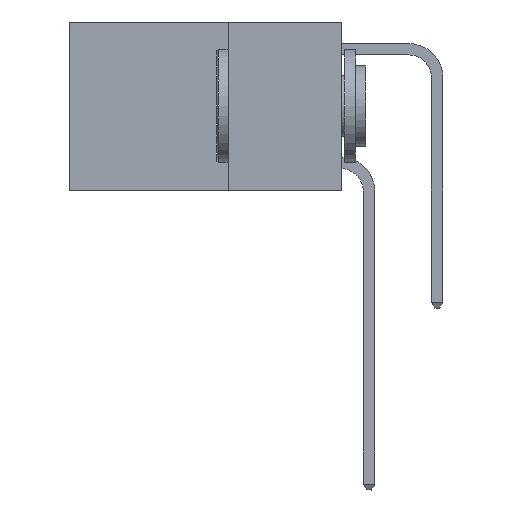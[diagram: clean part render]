
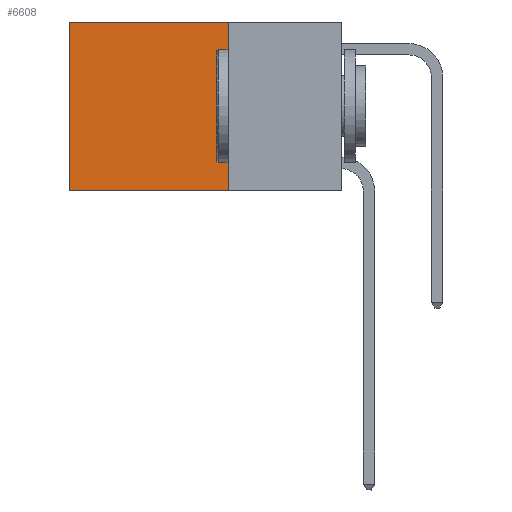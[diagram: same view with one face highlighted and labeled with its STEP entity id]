
A CAD part, left-side view. The second image highlights one B-rep face of the part: STEP entity #6608.
In plain terms, the highlighted planar face has unit normal (-1, 0, 0).
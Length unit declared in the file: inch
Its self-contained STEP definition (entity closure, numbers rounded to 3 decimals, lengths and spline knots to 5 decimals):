
#66 = CARTESIAN_POINT ( 'NONE',  ( 0.2625, 0.25, 0. ) ) ;
#132 = ORIENTED_EDGE ( 'NONE', *, *, #10196, .T. ) ;
#144 = CARTESIAN_POINT ( 'NONE',  ( 0.2625, 0.6, 0. ) ) ;
#981 = CARTESIAN_POINT ( 'NONE',  ( 0.2625, 0.6, 0. ) ) ;
#1362 = VECTOR ( 'NONE', #9491, 39.37008 ) ;
#1397 = DIRECTION ( 'NONE',  ( 1., 0., 0. ) ) ;
#1858 = VERTEX_POINT ( 'NONE', #144 ) ;
#1886 = LINE ( 'NONE', #7746, #2301 ) ;
#2301 = VECTOR ( 'NONE', #16773, 39.37008 ) ;
#2768 = CARTESIAN_POINT ( 'NONE',  ( 0.2625, 0.25, 0. ) ) ;
#4065 = LINE ( 'NONE', #981, #11034 ) ;
#4128 = ORIENTED_EDGE ( 'NONE', *, *, #5110, .F. ) ;
#5110 = EDGE_CURVE ( 'NONE', #11940, #6854, #1886, .T. ) ;
#6608 = ADVANCED_FACE ( 'NONE', ( #13193 ), #8014, .F. ) ;
#6854 = VERTEX_POINT ( 'NONE', #13717 ) ;
#7214 = ORIENTED_EDGE ( 'NONE', *, *, #8718, .F. ) ;
#7415 = CARTESIAN_POINT ( 'NONE',  ( 0.2625, 0.6, -0.37 ) ) ;
#7608 = ORIENTED_EDGE ( 'NONE', *, *, #11719, .T. ) ;
#7642 = VERTEX_POINT ( 'NONE', #7415 ) ;
#7746 = CARTESIAN_POINT ( 'NONE',  ( 0.2625, 0.25, 0. ) ) ;
#8014 = PLANE ( 'NONE',  #14003 ) ;
#8718 = EDGE_CURVE ( 'NONE', #6854, #7642, #12313, .T. ) ;
#9491 = DIRECTION ( 'NONE',  ( 0., 1., 0. ) ) ;
#10196 = EDGE_CURVE ( 'NONE', #1858, #7642, #4065, .T. ) ;
#10661 = DIRECTION ( 'NONE',  ( 0., 0., -1. ) ) ;
#11034 = VECTOR ( 'NONE', #16748, 39.37008 ) ;
#11230 = EDGE_LOOP ( 'NONE', ( #132, #7214, #4128, #7608 ) ) ;
#11602 = VECTOR ( 'NONE', #15844, 39.37008 ) ;
#11719 = EDGE_CURVE ( 'NONE', #11940, #1858, #12019, .T. ) ;
#11940 = VERTEX_POINT ( 'NONE', #16270 ) ;
#12019 = LINE ( 'NONE', #2768, #11602 ) ;
#12313 = LINE ( 'NONE', #15937, #1362 ) ;
#13193 = FACE_OUTER_BOUND ( 'NONE', #11230, .T. ) ;
#13717 = CARTESIAN_POINT ( 'NONE',  ( 0.2625, 0.25, -0.37 ) ) ;
#14003 = AXIS2_PLACEMENT_3D ( 'NONE', #66, #1397, #10661 ) ;
#15844 = DIRECTION ( 'NONE',  ( 0., 1., 0. ) ) ;
#15937 = CARTESIAN_POINT ( 'NONE',  ( 0.2625, 0.25, -0.37 ) ) ;
#16270 = CARTESIAN_POINT ( 'NONE',  ( 0.2625, 0.25, 0. ) ) ;
#16748 = DIRECTION ( 'NONE',  ( 0., 0., -1. ) ) ;
#16773 = DIRECTION ( 'NONE',  ( 0., 0., -1. ) ) ;
